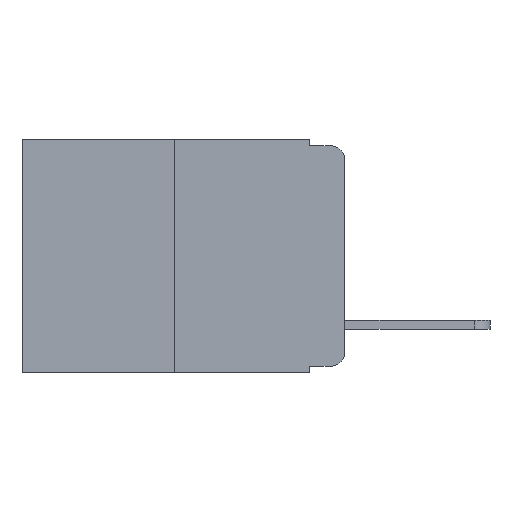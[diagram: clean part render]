
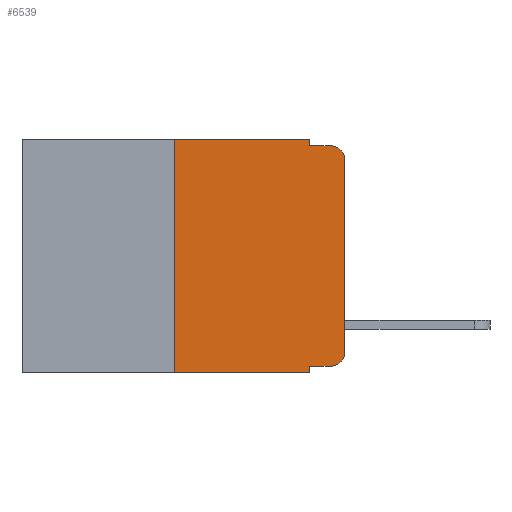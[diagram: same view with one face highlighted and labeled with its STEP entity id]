
A CAD part, left-side view. The second image highlights one B-rep face of the part: STEP entity #6539.
In plain terms, the highlighted planar face has unit normal (-1, 0, 0).
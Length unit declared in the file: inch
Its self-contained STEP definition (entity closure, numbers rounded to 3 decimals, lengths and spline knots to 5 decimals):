
#336 = VERTEX_POINT ( 'NONE', #6480 ) ;
#445 = CARTESIAN_POINT ( 'NONE',  ( 0., 0., -0.03 ) ) ;
#446 = EDGE_LOOP ( 'NONE', ( #517, #566, #609, #649, #749, #752, #784, #868, #979, #989 ) ) ;
#517 = ORIENTED_EDGE ( 'NONE', *, *, #3241, .T. ) ;
#566 = ORIENTED_EDGE ( 'NONE', *, *, #1904, .T. ) ;
#590 = VERTEX_POINT ( 'NONE', #1606 ) ;
#609 = ORIENTED_EDGE ( 'NONE', *, *, #6044, .F. ) ;
#649 = ORIENTED_EDGE ( 'NONE', *, *, #3883, .F. ) ;
#749 = ORIENTED_EDGE ( 'NONE', *, *, #2546, .F. ) ;
#752 = ORIENTED_EDGE ( 'NONE', *, *, #6458, .F. ) ;
#784 = ORIENTED_EDGE ( 'NONE', *, *, #6375, .T. ) ;
#847 = VERTEX_POINT ( 'NONE', #11437 ) ;
#868 = ORIENTED_EDGE ( 'NONE', *, *, #3349, .F. ) ;
#979 = ORIENTED_EDGE ( 'NONE', *, *, #6650, .T. ) ;
#989 = ORIENTED_EDGE ( 'NONE', *, *, #9492, .T. ) ;
#1272 = DIRECTION ( 'NONE',  ( 0., 0., -1. ) ) ;
#1546 = VERTEX_POINT ( 'NONE', #2889 ) ;
#1606 = CARTESIAN_POINT ( 'NONE',  ( 0., 0.25, 0. ) ) ;
#1672 = VERTEX_POINT ( 'NONE', #2854 ) ;
#1689 = VERTEX_POINT ( 'NONE', #6641 ) ;
#1719 = AXIS2_PLACEMENT_3D ( 'NONE', #9178, #9165, #9335 ) ;
#1904 = EDGE_CURVE ( 'NONE', #6196, #336, #9957, .T. ) ;
#2223 = VERTEX_POINT ( 'NONE', #11290 ) ;
#2546 = EDGE_CURVE ( 'NONE', #590, #2223, #4238, .T. ) ;
#2549 = CARTESIAN_POINT ( 'NONE',  ( 0., 0., 0. ) ) ;
#2706 = CARTESIAN_POINT ( 'NONE',  ( 0., 0., -0.313 ) ) ;
#2854 = CARTESIAN_POINT ( 'NONE',  ( 0., 0.051, -0.01 ) ) ;
#2889 = CARTESIAN_POINT ( 'NONE',  ( 0., 0.051, -0.333 ) ) ;
#3141 = VECTOR ( 'NONE', #11183, 39.37008 ) ;
#3241 = EDGE_CURVE ( 'NONE', #4843, #6196, #11371, .T. ) ;
#3349 = EDGE_CURVE ( 'NONE', #1546, #847, #9361, .T. ) ;
#3497 = LINE ( 'NONE', #6117, #3141 ) ;
#3566 = VERTEX_POINT ( 'NONE', #11098 ) ;
#3851 = LINE ( 'NONE', #5992, #6084 ) ;
#3883 = EDGE_CURVE ( 'NONE', #2223, #1672, #5265, .T. ) ;
#4169 = LINE ( 'NONE', #10073, #11036 ) ;
#4238 = LINE ( 'NONE', #10284, #4248 ) ;
#4248 = VECTOR ( 'NONE', #11137, 39.37008 ) ;
#4487 = AXIS2_PLACEMENT_3D ( 'NONE', #11025, #6692, #6680 ) ;
#4843 = VERTEX_POINT ( 'NONE', #2706 ) ;
#4857 = LINE ( 'NONE', #9565, #9226 ) ;
#5265 = LINE ( 'NONE', #10559, #6197 ) ;
#5992 = CARTESIAN_POINT ( 'NONE',  ( 0., 0.051, -0.333 ) ) ;
#6044 = EDGE_CURVE ( 'NONE', #1672, #336, #4169, .T. ) ;
#6073 = DIRECTION ( 'NONE',  ( 0., -1., 0. ) ) ;
#6084 = VECTOR ( 'NONE', #7521, 39.37008 ) ;
#6117 = CARTESIAN_POINT ( 'NONE',  ( 0., 0.473, -0.343 ) ) ;
#6196 = VERTEX_POINT ( 'NONE', #445 ) ;
#6197 = VECTOR ( 'NONE', #10814, 39.37008 ) ;
#6375 = EDGE_CURVE ( 'NONE', #3566, #847, #3497, .T. ) ;
#6458 = EDGE_CURVE ( 'NONE', #3566, #590, #4857, .T. ) ;
#6480 = CARTESIAN_POINT ( 'NONE',  ( 0., 0.02, -0.01 ) ) ;
#6539 = ADVANCED_FACE ( 'NONE', ( #7585 ), #11088, .F. ) ;
#6641 = CARTESIAN_POINT ( 'NONE',  ( 0., 0.02, -0.333 ) ) ;
#6650 = EDGE_CURVE ( 'NONE', #1546, #1689, #3851, .T. ) ;
#6680 = DIRECTION ( 'NONE',  ( 0., 0., -1. ) ) ;
#6692 = DIRECTION ( 'NONE',  ( 1., 0., 0. ) ) ;
#6900 = DIRECTION ( 'NONE',  ( 0., 0., -1. ) ) ;
#7219 = DIRECTION ( 'NONE',  ( 0., 0., 1. ) ) ;
#7521 = DIRECTION ( 'NONE',  ( 0., -1., 0. ) ) ;
#7585 = FACE_OUTER_BOUND ( 'NONE', #446, .T. ) ;
#9141 = VECTOR ( 'NONE', #1272, 39.37008 ) ;
#9165 = DIRECTION ( 'NONE',  ( -1., 0., 0. ) ) ;
#9178 = CARTESIAN_POINT ( 'NONE',  ( 0., 0.02, -0.313 ) ) ;
#9226 = VECTOR ( 'NONE', #7219, 39.37008 ) ;
#9335 = DIRECTION ( 'NONE',  ( 0., 0., -1. ) ) ;
#9361 = LINE ( 'NONE', #11854, #9141 ) ;
#9492 = EDGE_CURVE ( 'NONE', #1689, #4843, #11811, .T. ) ;
#9565 = CARTESIAN_POINT ( 'NONE',  ( 0., 0.25, 0. ) ) ;
#9600 = AXIS2_PLACEMENT_3D ( 'NONE', #10194, #10266, #6900 ) ;
#9957 = CIRCLE ( 'NONE', #9600, 0.02 ) ;
#10073 = CARTESIAN_POINT ( 'NONE',  ( 0., 0.051, -0.01 ) ) ;
#10194 = CARTESIAN_POINT ( 'NONE',  ( 0., 0.02, -0.03 ) ) ;
#10266 = DIRECTION ( 'NONE',  ( -1., 0., 0. ) ) ;
#10284 = CARTESIAN_POINT ( 'NONE',  ( 0., 0.473, 0. ) ) ;
#10559 = CARTESIAN_POINT ( 'NONE',  ( 0., 0.051, 0. ) ) ;
#10814 = DIRECTION ( 'NONE',  ( 0., 0., -1. ) ) ;
#11025 = CARTESIAN_POINT ( 'NONE',  ( 0., 0.473, 0. ) ) ;
#11036 = VECTOR ( 'NONE', #6073, 39.37008 ) ;
#11088 = PLANE ( 'NONE',  #4487 ) ;
#11098 = CARTESIAN_POINT ( 'NONE',  ( 0., 0.25, -0.343 ) ) ;
#11137 = DIRECTION ( 'NONE',  ( 0., -1., 0. ) ) ;
#11183 = DIRECTION ( 'NONE',  ( 0., -1., 0. ) ) ;
#11290 = CARTESIAN_POINT ( 'NONE',  ( 0., 0.051, 0. ) ) ;
#11312 = VECTOR ( 'NONE', #11915, 39.37008 ) ;
#11371 = LINE ( 'NONE', #2549, #11312 ) ;
#11437 = CARTESIAN_POINT ( 'NONE',  ( 0., 0.051, -0.343 ) ) ;
#11811 = CIRCLE ( 'NONE', #1719, 0.02 ) ;
#11854 = CARTESIAN_POINT ( 'NONE',  ( 0., 0.051, 0. ) ) ;
#11915 = DIRECTION ( 'NONE',  ( 0., 0., 1. ) ) ;
